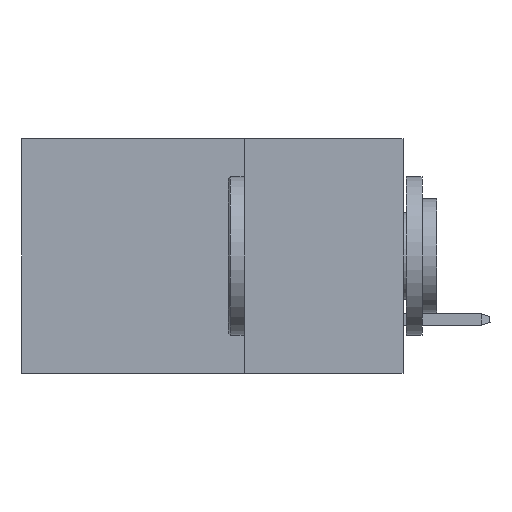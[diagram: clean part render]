
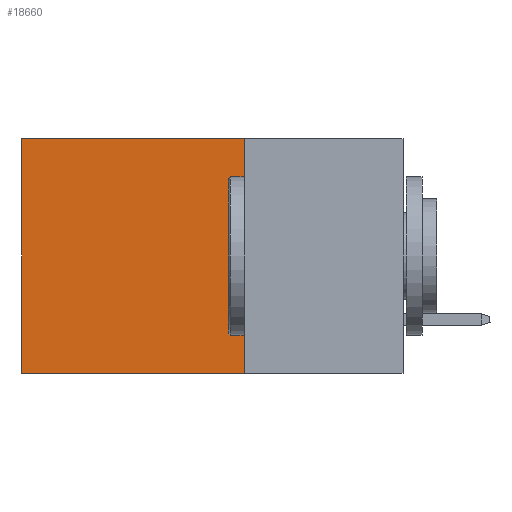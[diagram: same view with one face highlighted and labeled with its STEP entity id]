
A CAD part, left-side view. The second image highlights one B-rep face of the part: STEP entity #18660.
In plain terms, the highlighted planar face has unit normal (-1, 0, 0).
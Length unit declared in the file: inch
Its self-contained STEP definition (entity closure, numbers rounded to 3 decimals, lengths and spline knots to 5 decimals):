
#289 = AXIS2_PLACEMENT_3D ( 'NONE', #2060, #8621, #353 ) ;
#314 = CARTESIAN_POINT ( 'NONE',  ( 0.2875, 0.25, -0.37 ) ) ;
#353 = DIRECTION ( 'NONE',  ( 0., 0., -1. ) ) ;
#840 = LINE ( 'NONE', #7172, #3449 ) ;
#1152 = EDGE_CURVE ( 'NONE', #20814, #8016, #840, .T. ) ;
#1472 = CARTESIAN_POINT ( 'NONE',  ( 0.2875, 0.6, 0. ) ) ;
#2060 = CARTESIAN_POINT ( 'NONE',  ( 0.2875, 0.25, 0. ) ) ;
#2989 = EDGE_CURVE ( 'NONE', #15511, #4822, #16510, .T. ) ;
#3449 = VECTOR ( 'NONE', #15526, 39.37008 ) ;
#3478 = VECTOR ( 'NONE', #5037, 39.37008 ) ;
#4822 = VERTEX_POINT ( 'NONE', #6169 ) ;
#5037 = DIRECTION ( 'NONE',  ( 0., 1., 0. ) ) ;
#6051 = EDGE_CURVE ( 'NONE', #8016, #4822, #14820, .T. ) ;
#6169 = CARTESIAN_POINT ( 'NONE',  ( 0.2875, 0.6, -0.37 ) ) ;
#7172 = CARTESIAN_POINT ( 'NONE',  ( 0.2875, 0.25, 0. ) ) ;
#7794 = CARTESIAN_POINT ( 'NONE',  ( 0.2875, 0.25, 0. ) ) ;
#7977 = ORIENTED_EDGE ( 'NONE', *, *, #6051, .T. ) ;
#7989 = LINE ( 'NONE', #12831, #9423 ) ;
#8016 = VERTEX_POINT ( 'NONE', #1472 ) ;
#8621 = DIRECTION ( 'NONE',  ( 1., 0., 0. ) ) ;
#9121 = ORIENTED_EDGE ( 'NONE', *, *, #2989, .F. ) ;
#9423 = VECTOR ( 'NONE', #13154, 39.37008 ) ;
#10144 = PLANE ( 'NONE',  #289 ) ;
#11112 = VECTOR ( 'NONE', #18230, 39.37008 ) ;
#11641 = CARTESIAN_POINT ( 'NONE',  ( 0.2875, 0.6, 0. ) ) ;
#12562 = EDGE_CURVE ( 'NONE', #20814, #15511, #7989, .T. ) ;
#12831 = CARTESIAN_POINT ( 'NONE',  ( 0.2875, 0.25, 0. ) ) ;
#13154 = DIRECTION ( 'NONE',  ( 0., 0., -1. ) ) ;
#14820 = LINE ( 'NONE', #11641, #11112 ) ;
#15436 = ORIENTED_EDGE ( 'NONE', *, *, #1152, .T. ) ;
#15511 = VERTEX_POINT ( 'NONE', #20154 ) ;
#15526 = DIRECTION ( 'NONE',  ( 0., 1., 0. ) ) ;
#16510 = LINE ( 'NONE', #314, #3478 ) ;
#18056 = ORIENTED_EDGE ( 'NONE', *, *, #12562, .F. ) ;
#18230 = DIRECTION ( 'NONE',  ( 0., 0., -1. ) ) ;
#18346 = FACE_OUTER_BOUND ( 'NONE', #20396, .T. ) ;
#18660 = ADVANCED_FACE ( 'NONE', ( #18346 ), #10144, .F. ) ;
#20154 = CARTESIAN_POINT ( 'NONE',  ( 0.2875, 0.25, -0.37 ) ) ;
#20396 = EDGE_LOOP ( 'NONE', ( #7977, #9121, #18056, #15436 ) ) ;
#20814 = VERTEX_POINT ( 'NONE', #7794 ) ;
